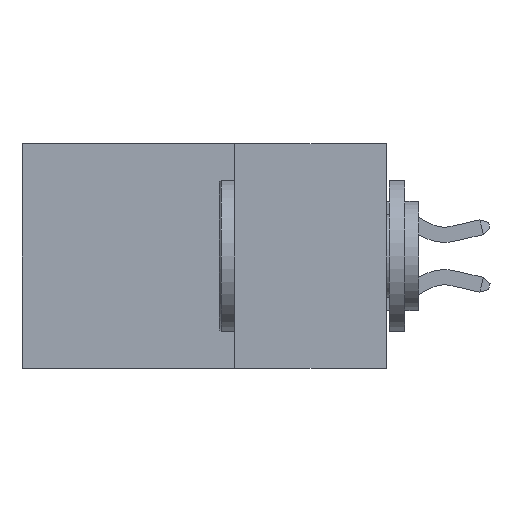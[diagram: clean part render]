
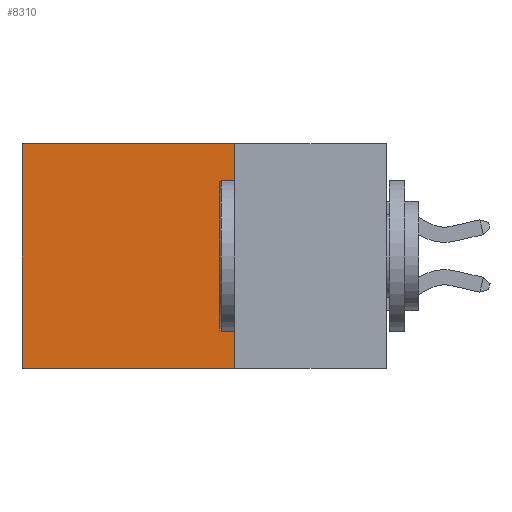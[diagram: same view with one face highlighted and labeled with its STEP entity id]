
A CAD part, left-side view. The second image highlights one B-rep face of the part: STEP entity #8310.
In plain terms, the highlighted planar face has unit normal (-1, 0, 0).
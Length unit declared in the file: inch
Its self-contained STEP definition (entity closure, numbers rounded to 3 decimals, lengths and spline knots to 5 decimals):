
#60 = DIRECTION ( 'NONE',  ( 0., 0., -1. ) ) ;
#416 = CARTESIAN_POINT ( 'NONE',  ( 0.2615, 0.25, -0.37 ) ) ;
#1201 = ORIENTED_EDGE ( 'NONE', *, *, #9139, .F. ) ;
#1421 = CARTESIAN_POINT ( 'NONE',  ( 0.2615, 0.6, 0. ) ) ;
#1836 = DIRECTION ( 'NONE',  ( 1., 0., 0. ) ) ;
#2511 = LINE ( 'NONE', #14925, #9591 ) ;
#4675 = VECTOR ( 'NONE', #60, 39.37008 ) ;
#5459 = AXIS2_PLACEMENT_3D ( 'NONE', #416, #1836, #11753 ) ;
#6062 = ORIENTED_EDGE ( 'NONE', *, *, #15804, .T. ) ;
#6535 = DIRECTION ( 'NONE',  ( 0., 1., 0. ) ) ;
#8310 = ADVANCED_FACE ( 'NONE', ( #12988 ), #8895, .F. ) ;
#8407 = LINE ( 'NONE', #14170, #4675 ) ;
#8562 = CARTESIAN_POINT ( 'NONE',  ( 0.2615, 0.25, -0.37 ) ) ;
#8895 = PLANE ( 'NONE',  #5459 ) ;
#9019 = LINE ( 'NONE', #8562, #15995 ) ;
#9139 = EDGE_CURVE ( 'NONE', #9507, #16223, #9019, .T. ) ;
#9214 = DIRECTION ( 'NONE',  ( 0., 0., -1. ) ) ;
#9424 = CARTESIAN_POINT ( 'NONE',  ( 0.2615, 0.25, -0.37 ) ) ;
#9507 = VERTEX_POINT ( 'NONE', #9424 ) ;
#9591 = VECTOR ( 'NONE', #6535, 39.37008 ) ;
#9983 = DIRECTION ( 'NONE',  ( 0., 1., 0. ) ) ;
#10682 = LINE ( 'NONE', #17531, #15239 ) ;
#11753 = DIRECTION ( 'NONE',  ( 0., 0., -1. ) ) ;
#12008 = EDGE_CURVE ( 'NONE', #14837, #14296, #2511, .T. ) ;
#12337 = CARTESIAN_POINT ( 'NONE',  ( 0.2615, 0.25, 0. ) ) ;
#12788 = ORIENTED_EDGE ( 'NONE', *, *, #16870, .F. ) ;
#12988 = FACE_OUTER_BOUND ( 'NONE', #15490, .T. ) ;
#14170 = CARTESIAN_POINT ( 'NONE',  ( 0.2615, 0.25, -0.37 ) ) ;
#14296 = VERTEX_POINT ( 'NONE', #1421 ) ;
#14837 = VERTEX_POINT ( 'NONE', #12337 ) ;
#14925 = CARTESIAN_POINT ( 'NONE',  ( 0.2615, 0.25, 0. ) ) ;
#15239 = VECTOR ( 'NONE', #9214, 39.37008 ) ;
#15490 = EDGE_LOOP ( 'NONE', ( #6062, #1201, #12788, #17029 ) ) ;
#15531 = CARTESIAN_POINT ( 'NONE',  ( 0.2615, 0.6, -0.37 ) ) ;
#15804 = EDGE_CURVE ( 'NONE', #14296, #16223, #10682, .T. ) ;
#15995 = VECTOR ( 'NONE', #9983, 39.37008 ) ;
#16223 = VERTEX_POINT ( 'NONE', #15531 ) ;
#16870 = EDGE_CURVE ( 'NONE', #14837, #9507, #8407, .T. ) ;
#17029 = ORIENTED_EDGE ( 'NONE', *, *, #12008, .T. ) ;
#17531 = CARTESIAN_POINT ( 'NONE',  ( 0.2615, 0.6, -0.37 ) ) ;
